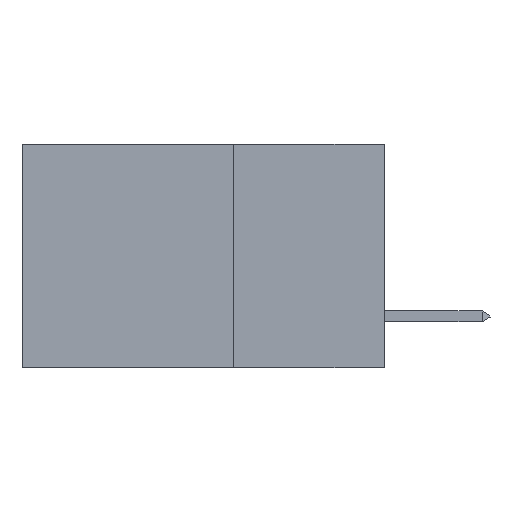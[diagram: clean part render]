
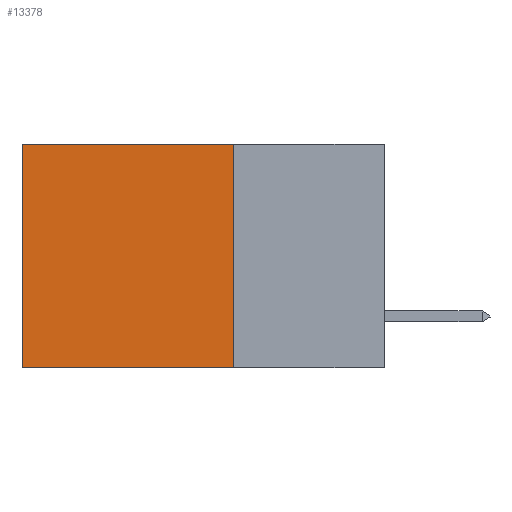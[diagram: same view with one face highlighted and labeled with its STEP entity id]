
A CAD part, left-side view. The second image highlights one B-rep face of the part: STEP entity #13378.
In plain terms, the highlighted planar face has unit normal (-1, 0, 0).
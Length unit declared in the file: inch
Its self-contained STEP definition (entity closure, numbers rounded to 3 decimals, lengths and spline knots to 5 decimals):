
#208 = EDGE_CURVE ( 'NONE', #19428, #24729, #21390, .T. ) ;
#1010 = ORIENTED_EDGE ( 'NONE', *, *, #4705, .T. ) ;
#1093 = FACE_OUTER_BOUND ( 'NONE', #4347, .T. ) ;
#1216 = CARTESIAN_POINT ( 'NONE',  ( 0.2875, 0.25, 0. ) ) ;
#1544 = ORIENTED_EDGE ( 'NONE', *, *, #22953, .F. ) ;
#1782 = LINE ( 'NONE', #22964, #14395 ) ;
#2235 = VECTOR ( 'NONE', #4636, 39.37008 ) ;
#4347 = EDGE_LOOP ( 'NONE', ( #1010, #6662, #1544, #23360 ) ) ;
#4636 = DIRECTION ( 'NONE',  ( 0., 0., -1. ) ) ;
#4705 = EDGE_CURVE ( 'NONE', #11562, #24729, #24759, .T. ) ;
#4771 = AXIS2_PLACEMENT_3D ( 'NONE', #1216, #24059, #6924 ) ;
#6057 = VECTOR ( 'NONE', #19954, 39.37008 ) ;
#6662 = ORIENTED_EDGE ( 'NONE', *, *, #208, .F. ) ;
#6924 = DIRECTION ( 'NONE',  ( 0., 0., -1. ) ) ;
#9421 = DIRECTION ( 'NONE',  ( 0., 1., 0. ) ) ;
#10680 = PLANE ( 'NONE',  #4771 ) ;
#11562 = VERTEX_POINT ( 'NONE', #19614 ) ;
#13114 = CARTESIAN_POINT ( 'NONE',  ( 0.2875, 0.25, -0.37 ) ) ;
#13378 = ADVANCED_FACE ( 'NONE', ( #1093 ), #10680, .F. ) ;
#14395 = VECTOR ( 'NONE', #9421, 39.37008 ) ;
#14522 = CARTESIAN_POINT ( 'NONE',  ( 0.2875, 0.6, 0. ) ) ;
#15366 = VECTOR ( 'NONE', #20436, 39.37008 ) ;
#17486 = LINE ( 'NONE', #23955, #15366 ) ;
#18018 = CARTESIAN_POINT ( 'NONE',  ( 0.2875, 0.25, -0.37 ) ) ;
#18505 = EDGE_CURVE ( 'NONE', #24301, #11562, #1782, .T. ) ;
#18682 = CARTESIAN_POINT ( 'NONE',  ( 0.2875, 0.25, 0. ) ) ;
#19428 = VERTEX_POINT ( 'NONE', #13114 ) ;
#19614 = CARTESIAN_POINT ( 'NONE',  ( 0.2875, 0.6, 0. ) ) ;
#19954 = DIRECTION ( 'NONE',  ( 0., 1., 0. ) ) ;
#20436 = DIRECTION ( 'NONE',  ( 0., 0., -1. ) ) ;
#21390 = LINE ( 'NONE', #18018, #6057 ) ;
#22309 = CARTESIAN_POINT ( 'NONE',  ( 0.2875, 0.6, -0.37 ) ) ;
#22953 = EDGE_CURVE ( 'NONE', #24301, #19428, #17486, .T. ) ;
#22964 = CARTESIAN_POINT ( 'NONE',  ( 0.2875, 0.25, 0. ) ) ;
#23360 = ORIENTED_EDGE ( 'NONE', *, *, #18505, .T. ) ;
#23955 = CARTESIAN_POINT ( 'NONE',  ( 0.2875, 0.25, 0. ) ) ;
#24059 = DIRECTION ( 'NONE',  ( 1., 0., 0. ) ) ;
#24301 = VERTEX_POINT ( 'NONE', #18682 ) ;
#24729 = VERTEX_POINT ( 'NONE', #22309 ) ;
#24759 = LINE ( 'NONE', #14522, #2235 ) ;
